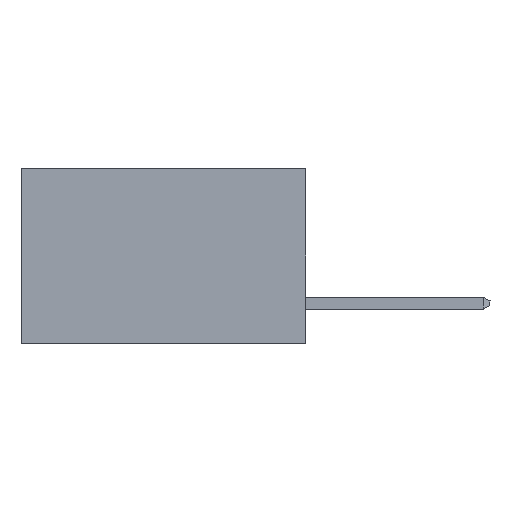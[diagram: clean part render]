
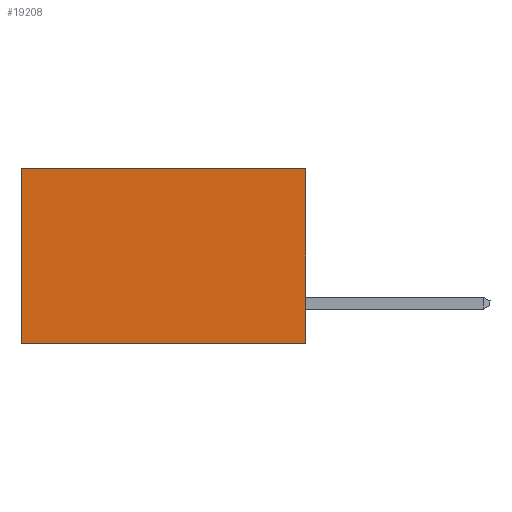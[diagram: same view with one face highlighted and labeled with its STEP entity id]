
A CAD part, left-side view. The second image highlights one B-rep face of the part: STEP entity #19208.
In plain terms, the highlighted planar face has unit normal (-1, 0, 0).
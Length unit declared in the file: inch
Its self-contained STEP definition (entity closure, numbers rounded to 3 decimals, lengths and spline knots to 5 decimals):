
#63 = DIRECTION ( 'NONE',  ( 0., 0., -1. ) ) ;
#1282 = DIRECTION ( 'NONE',  ( 0., 0., -1. ) ) ;
#2465 = VERTEX_POINT ( 'NONE', #6630 ) ;
#3292 = VERTEX_POINT ( 'NONE', #22269 ) ;
#3331 = EDGE_CURVE ( 'NONE', #3292, #2465, #8125, .T. ) ;
#3591 = ORIENTED_EDGE ( 'NONE', *, *, #21433, .T. ) ;
#3628 = CARTESIAN_POINT ( 'NONE',  ( 0.298, 0., 0. ) ) ;
#4310 = LINE ( 'NONE', #18591, #21950 ) ;
#5320 = DIRECTION ( 'NONE',  ( 1., 0., 0. ) ) ;
#6105 = VERTEX_POINT ( 'NONE', #20344 ) ;
#6452 = VECTOR ( 'NONE', #63, 39.37008 ) ;
#6630 = CARTESIAN_POINT ( 'NONE',  ( 0.298, 0.6, 0. ) ) ;
#7604 = ORIENTED_EDGE ( 'NONE', *, *, #12488, .F. ) ;
#8105 = VECTOR ( 'NONE', #10112, 39.37008 ) ;
#8125 = LINE ( 'NONE', #13820, #8105 ) ;
#8548 = VERTEX_POINT ( 'NONE', #20694 ) ;
#9089 = CARTESIAN_POINT ( 'NONE',  ( 0.298, 0.6, 0. ) ) ;
#9573 = LINE ( 'NONE', #9089, #6452 ) ;
#10112 = DIRECTION ( 'NONE',  ( 0., 1., 0. ) ) ;
#11625 = FACE_OUTER_BOUND ( 'NONE', #12681, .T. ) ;
#12488 = EDGE_CURVE ( 'NONE', #6105, #8548, #4310, .T. ) ;
#12681 = EDGE_LOOP ( 'NONE', ( #3591, #7604, #14148, #17178 ) ) ;
#13735 = CARTESIAN_POINT ( 'NONE',  ( 0.298, 0., 0. ) ) ;
#13820 = CARTESIAN_POINT ( 'NONE',  ( 0.298, 0., 0. ) ) ;
#14148 = ORIENTED_EDGE ( 'NONE', *, *, #18560, .F. ) ;
#14320 = DIRECTION ( 'NONE',  ( 0., 0., -1. ) ) ;
#15462 = DIRECTION ( 'NONE',  ( 0., 1., 0. ) ) ;
#16506 = LINE ( 'NONE', #13735, #19610 ) ;
#17178 = ORIENTED_EDGE ( 'NONE', *, *, #3331, .T. ) ;
#18560 = EDGE_CURVE ( 'NONE', #3292, #6105, #16506, .T. ) ;
#18591 = CARTESIAN_POINT ( 'NONE',  ( 0.298, 0., -0.37 ) ) ;
#19208 = ADVANCED_FACE ( 'NONE', ( #11625 ), #20165, .F. ) ;
#19610 = VECTOR ( 'NONE', #1282, 39.37008 ) ;
#20165 = PLANE ( 'NONE',  #21675 ) ;
#20344 = CARTESIAN_POINT ( 'NONE',  ( 0.298, 0., -0.37 ) ) ;
#20694 = CARTESIAN_POINT ( 'NONE',  ( 0.298, 0.6, -0.37 ) ) ;
#21433 = EDGE_CURVE ( 'NONE', #2465, #8548, #9573, .T. ) ;
#21675 = AXIS2_PLACEMENT_3D ( 'NONE', #3628, #5320, #14320 ) ;
#21950 = VECTOR ( 'NONE', #15462, 39.37008 ) ;
#22269 = CARTESIAN_POINT ( 'NONE',  ( 0.298, 0., 0. ) ) ;
